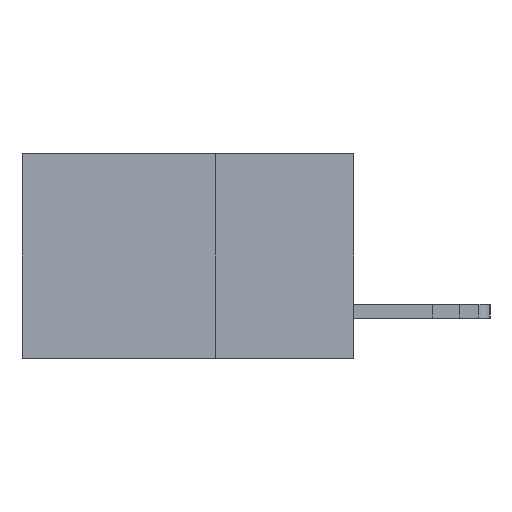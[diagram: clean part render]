
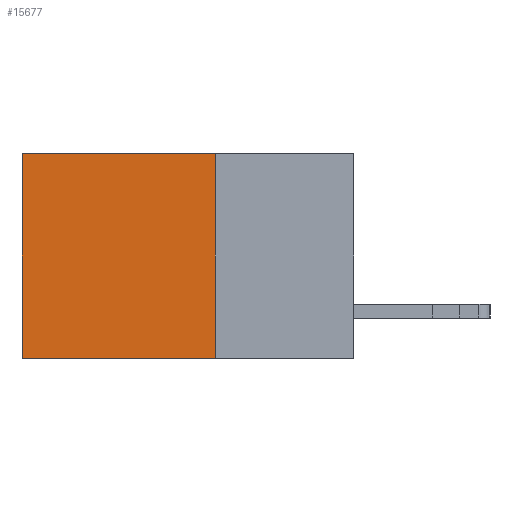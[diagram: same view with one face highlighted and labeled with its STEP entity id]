
A CAD part, left-side view. The second image highlights one B-rep face of the part: STEP entity #15677.
In plain terms, the highlighted planar face has unit normal (-1, 0, 0).
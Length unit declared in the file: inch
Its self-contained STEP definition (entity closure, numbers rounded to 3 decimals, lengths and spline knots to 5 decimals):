
#753 = VECTOR ( 'NONE', #17706, 39.37008 ) ;
#1915 = VERTEX_POINT ( 'NONE', #15516 ) ;
#2285 = CARTESIAN_POINT ( 'NONE',  ( 0.2875, 0.25, 0. ) ) ;
#2377 = ORIENTED_EDGE ( 'NONE', *, *, #17844, .T. ) ;
#3252 = LINE ( 'NONE', #7869, #12212 ) ;
#3563 = CARTESIAN_POINT ( 'NONE',  ( 0.2875, 0.25, -0.37 ) ) ;
#4137 = DIRECTION ( 'NONE',  ( 1., 0., 0. ) ) ;
#4612 = CARTESIAN_POINT ( 'NONE',  ( 0.2875, 0.25, 0. ) ) ;
#5567 = FACE_OUTER_BOUND ( 'NONE', #14199, .T. ) ;
#6184 = VERTEX_POINT ( 'NONE', #7981 ) ;
#6235 = ORIENTED_EDGE ( 'NONE', *, *, #9198, .F. ) ;
#6433 = VERTEX_POINT ( 'NONE', #14815 ) ;
#7138 = LINE ( 'NONE', #9969, #753 ) ;
#7489 = DIRECTION ( 'NONE',  ( 0., 0., -1. ) ) ;
#7869 = CARTESIAN_POINT ( 'NONE',  ( 0.2875, 0.6, 0. ) ) ;
#7981 = CARTESIAN_POINT ( 'NONE',  ( 0.2875, 0.25, -0.37 ) ) ;
#9198 = EDGE_CURVE ( 'NONE', #6184, #1915, #9537, .T. ) ;
#9325 = VECTOR ( 'NONE', #12385, 39.37008 ) ;
#9423 = DIRECTION ( 'NONE',  ( 0., 0., -1. ) ) ;
#9537 = LINE ( 'NONE', #3563, #9325 ) ;
#9706 = ORIENTED_EDGE ( 'NONE', *, *, #17559, .F. ) ;
#9969 = CARTESIAN_POINT ( 'NONE',  ( 0.2875, 0.25, 0. ) ) ;
#11281 = VECTOR ( 'NONE', #7489, 39.37008 ) ;
#11589 = AXIS2_PLACEMENT_3D ( 'NONE', #11808, #4137, #12990 ) ;
#11808 = CARTESIAN_POINT ( 'NONE',  ( 0.2875, 0.25, 0. ) ) ;
#12212 = VECTOR ( 'NONE', #9423, 39.37008 ) ;
#12385 = DIRECTION ( 'NONE',  ( 0., 1., 0. ) ) ;
#12565 = VERTEX_POINT ( 'NONE', #2285 ) ;
#12990 = DIRECTION ( 'NONE',  ( 0., 0., -1. ) ) ;
#13088 = PLANE ( 'NONE',  #11589 ) ;
#14199 = EDGE_LOOP ( 'NONE', ( #2377, #6235, #9706, #17577 ) ) ;
#14815 = CARTESIAN_POINT ( 'NONE',  ( 0.2875, 0.6, 0. ) ) ;
#15516 = CARTESIAN_POINT ( 'NONE',  ( 0.2875, 0.6, -0.37 ) ) ;
#15677 = ADVANCED_FACE ( 'NONE', ( #5567 ), #13088, .F. ) ;
#17559 = EDGE_CURVE ( 'NONE', #12565, #6184, #17889, .T. ) ;
#17577 = ORIENTED_EDGE ( 'NONE', *, *, #18549, .T. ) ;
#17706 = DIRECTION ( 'NONE',  ( 0., 1., 0. ) ) ;
#17844 = EDGE_CURVE ( 'NONE', #6433, #1915, #3252, .T. ) ;
#17889 = LINE ( 'NONE', #4612, #11281 ) ;
#18549 = EDGE_CURVE ( 'NONE', #12565, #6433, #7138, .T. ) ;
